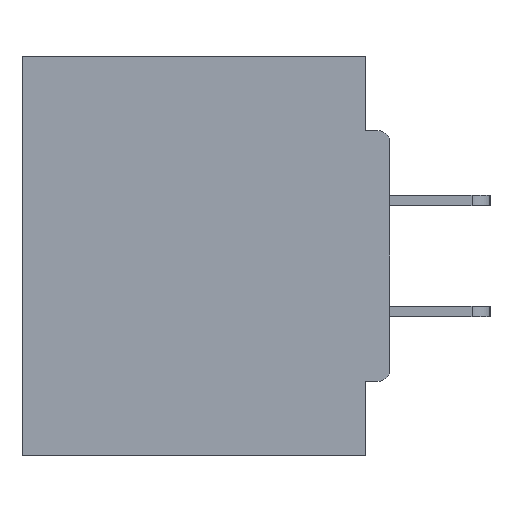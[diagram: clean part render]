
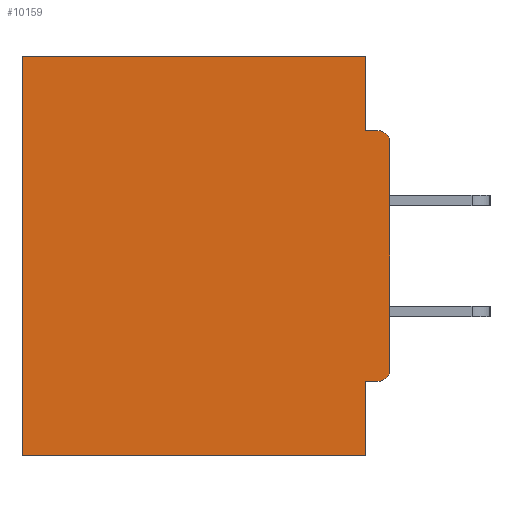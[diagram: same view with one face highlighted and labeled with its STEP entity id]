
A CAD part, left-side view. The second image highlights one B-rep face of the part: STEP entity #10159.
In plain terms, the highlighted planar face has unit normal (-1, 0, 0).
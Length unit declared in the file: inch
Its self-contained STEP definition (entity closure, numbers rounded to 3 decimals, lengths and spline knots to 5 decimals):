
#794 = VERTEX_POINT ( 'NONE', #20351 ) ;
#1736 = VECTOR ( 'NONE', #23781, 39.37008 ) ;
#2145 = CARTESIAN_POINT ( 'NONE',  ( 0.298, 0.031, 0. ) ) ;
#2323 = LINE ( 'NONE', #31143, #29455 ) ;
#2395 = ORIENTED_EDGE ( 'NONE', *, *, #12134, .T. ) ;
#2410 = LINE ( 'NONE', #11653, #31102 ) ;
#2891 = CARTESIAN_POINT ( 'NONE',  ( 0.298, 0.46, 0. ) ) ;
#3004 = VECTOR ( 'NONE', #20226, 39.37008 ) ;
#3112 = CARTESIAN_POINT ( 'NONE',  ( 0.298, 0.031, -0.4065 ) ) ;
#3311 = ORIENTED_EDGE ( 'NONE', *, *, #6204, .T. ) ;
#3336 = EDGE_CURVE ( 'NONE', #17227, #13647, #30037, .T. ) ;
#4221 = LINE ( 'NONE', #14068, #24120 ) ;
#4267 = ORIENTED_EDGE ( 'NONE', *, *, #30350, .F. ) ;
#4482 = DIRECTION ( 'NONE',  ( 0., 0., -1. ) ) ;
#4866 = ORIENTED_EDGE ( 'NONE', *, *, #8828, .F. ) ;
#5193 = DIRECTION ( 'NONE',  ( 0., 0., -1. ) ) ;
#5546 = DIRECTION ( 'NONE',  ( -1., 0., 0. ) ) ;
#5836 = FACE_OUTER_BOUND ( 'NONE', #11974, .T. ) ;
#6204 = EDGE_CURVE ( 'NONE', #23415, #15420, #2323, .T. ) ;
#6659 = CARTESIAN_POINT ( 'NONE',  ( 0.298, 0., -0.4065 ) ) ;
#7043 = CARTESIAN_POINT ( 'NONE',  ( 0.298, 0.031, -0.0935 ) ) ;
#7127 = EDGE_CURVE ( 'NONE', #23415, #31194, #7579, .T. ) ;
#7579 = LINE ( 'NONE', #20417, #12535 ) ;
#7603 = EDGE_CURVE ( 'NONE', #10966, #13647, #27833, .T. ) ;
#7624 = LINE ( 'NONE', #18329, #3004 ) ;
#8681 = CARTESIAN_POINT ( 'NONE',  ( 0.298, 0., 0. ) ) ;
#8828 = EDGE_CURVE ( 'NONE', #31194, #24669, #18188, .T. ) ;
#8875 = CARTESIAN_POINT ( 'NONE',  ( 0.298, 0.015, -0.1085 ) ) ;
#9364 = ORIENTED_EDGE ( 'NONE', *, *, #17234, .F. ) ;
#9815 = ORIENTED_EDGE ( 'NONE', *, *, #11497, .F. ) ;
#10159 = ADVANCED_FACE ( 'NONE', ( #5836 ), #30802, .F. ) ;
#10211 = VECTOR ( 'NONE', #24678, 39.37008 ) ;
#10332 = VERTEX_POINT ( 'NONE', #3112 ) ;
#10966 = VERTEX_POINT ( 'NONE', #12549 ) ;
#11131 = ORIENTED_EDGE ( 'NONE', *, *, #7603, .F. ) ;
#11497 = EDGE_CURVE ( 'NONE', #10332, #19063, #4221, .T. ) ;
#11653 = CARTESIAN_POINT ( 'NONE',  ( 0.298, 0.46, 0. ) ) ;
#11974 = EDGE_LOOP ( 'NONE', ( #2395, #4866, #14590, #3311, #15542, #9364, #9815, #4267, #21989, #11131 ) ) ;
#12134 = EDGE_CURVE ( 'NONE', #10966, #24669, #19498, .T. ) ;
#12202 = AXIS2_PLACEMENT_3D ( 'NONE', #15364, #5546, #13203 ) ;
#12535 = VECTOR ( 'NONE', #23085, 39.37008 ) ;
#12549 = CARTESIAN_POINT ( 'NONE',  ( 0.298, 0., -0.1085 ) ) ;
#13203 = DIRECTION ( 'NONE',  ( 0., 0., -1. ) ) ;
#13587 = DIRECTION ( 'NONE',  ( 0., 1., 0. ) ) ;
#13647 = VERTEX_POINT ( 'NONE', #22661 ) ;
#14068 = CARTESIAN_POINT ( 'NONE',  ( 0.298, 0.031, -0.5 ) ) ;
#14356 = EDGE_CURVE ( 'NONE', #15420, #794, #2410, .T. ) ;
#14590 = ORIENTED_EDGE ( 'NONE', *, *, #7127, .F. ) ;
#15364 = CARTESIAN_POINT ( 'NONE',  ( 0.298, 0.015, -0.3915 ) ) ;
#15420 = VERTEX_POINT ( 'NONE', #2891 ) ;
#15542 = ORIENTED_EDGE ( 'NONE', *, *, #14356, .T. ) ;
#15846 = AXIS2_PLACEMENT_3D ( 'NONE', #8875, #18967, #26031 ) ;
#17227 = VERTEX_POINT ( 'NONE', #30123 ) ;
#17234 = EDGE_CURVE ( 'NONE', #19063, #794, #7624, .T. ) ;
#18188 = LINE ( 'NONE', #28008, #29253 ) ;
#18329 = CARTESIAN_POINT ( 'NONE',  ( 0.298, 0., -0.5 ) ) ;
#18967 = DIRECTION ( 'NONE',  ( -1., 0., 0. ) ) ;
#18983 = LINE ( 'NONE', #6659, #1736 ) ;
#19063 = VERTEX_POINT ( 'NONE', #20785 ) ;
#19498 = CIRCLE ( 'NONE', #15846, 0.015 ) ;
#20226 = DIRECTION ( 'NONE',  ( 0., 1., 0. ) ) ;
#20351 = CARTESIAN_POINT ( 'NONE',  ( 0.298, 0.46, -0.5 ) ) ;
#20417 = CARTESIAN_POINT ( 'NONE',  ( 0.298, 0.031, -0.5 ) ) ;
#20785 = CARTESIAN_POINT ( 'NONE',  ( 0.298, 0.031, -0.5 ) ) ;
#21989 = ORIENTED_EDGE ( 'NONE', *, *, #3336, .T. ) ;
#22661 = CARTESIAN_POINT ( 'NONE',  ( 0.298, 0., -0.3915 ) ) ;
#23085 = DIRECTION ( 'NONE',  ( 0., 0., -1. ) ) ;
#23415 = VERTEX_POINT ( 'NONE', #2145 ) ;
#23781 = DIRECTION ( 'NONE',  ( 0., 1., 0. ) ) ;
#24120 = VECTOR ( 'NONE', #5193, 39.37008 ) ;
#24669 = VERTEX_POINT ( 'NONE', #25194 ) ;
#24678 = DIRECTION ( 'NONE',  ( 0., 0., -1. ) ) ;
#25194 = CARTESIAN_POINT ( 'NONE',  ( 0.298, 0.015, -0.0935 ) ) ;
#25846 = DIRECTION ( 'NONE',  ( 0., 0., -1. ) ) ;
#26031 = DIRECTION ( 'NONE',  ( 0., 0., -1. ) ) ;
#26705 = DIRECTION ( 'NONE',  ( 1., 0., 0. ) ) ;
#27833 = LINE ( 'NONE', #29449, #10211 ) ;
#28008 = CARTESIAN_POINT ( 'NONE',  ( 0.298, 0., -0.0935 ) ) ;
#28313 = DIRECTION ( 'NONE',  ( 0., -1., 0. ) ) ;
#29253 = VECTOR ( 'NONE', #28313, 39.37008 ) ;
#29449 = CARTESIAN_POINT ( 'NONE',  ( 0.298, 0., 0. ) ) ;
#29455 = VECTOR ( 'NONE', #13587, 39.37008 ) ;
#30037 = CIRCLE ( 'NONE', #12202, 0.015 ) ;
#30123 = CARTESIAN_POINT ( 'NONE',  ( 0.298, 0.015, -0.4065 ) ) ;
#30350 = EDGE_CURVE ( 'NONE', #17227, #10332, #18983, .T. ) ;
#30550 = AXIS2_PLACEMENT_3D ( 'NONE', #8681, #26705, #25846 ) ;
#30802 = PLANE ( 'NONE',  #30550 ) ;
#31102 = VECTOR ( 'NONE', #4482, 39.37008 ) ;
#31143 = CARTESIAN_POINT ( 'NONE',  ( 0.298, 0., 0. ) ) ;
#31194 = VERTEX_POINT ( 'NONE', #7043 ) ;
